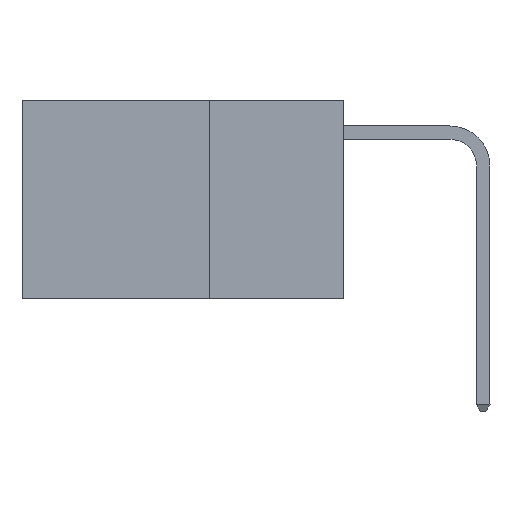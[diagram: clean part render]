
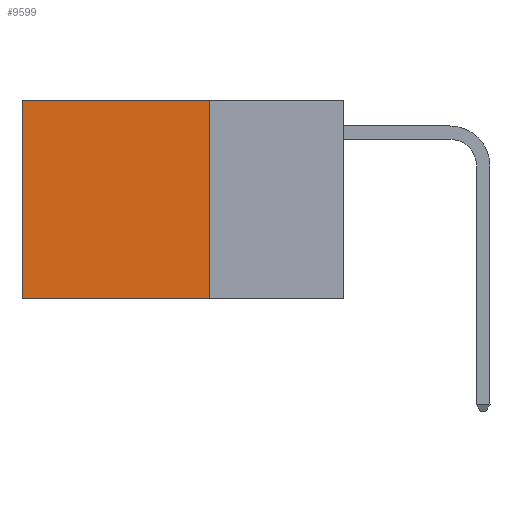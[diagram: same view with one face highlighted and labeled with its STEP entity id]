
A CAD part, left-side view. The second image highlights one B-rep face of the part: STEP entity #9599.
In plain terms, the highlighted planar face has unit normal (-1, 0, 0).
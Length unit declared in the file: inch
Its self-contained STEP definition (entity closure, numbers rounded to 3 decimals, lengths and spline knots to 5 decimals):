
#160 = DIRECTION ( 'NONE',  ( 1., 0., 0. ) ) ;
#245 = VERTEX_POINT ( 'NONE', #9115 ) ;
#525 = CARTESIAN_POINT ( 'NONE',  ( 0.2625, 0.25, -0.37 ) ) ;
#657 = LINE ( 'NONE', #6337, #13990 ) ;
#800 = ORIENTED_EDGE ( 'NONE', *, *, #7438, .F. ) ;
#882 = VECTOR ( 'NONE', #3667, 39.37008 ) ;
#1058 = LINE ( 'NONE', #10226, #7920 ) ;
#1060 = VERTEX_POINT ( 'NONE', #13839 ) ;
#1186 = CARTESIAN_POINT ( 'NONE',  ( 0.2625, 0.6, -0.37 ) ) ;
#1556 = ORIENTED_EDGE ( 'NONE', *, *, #12835, .F. ) ;
#3667 = DIRECTION ( 'NONE',  ( 0., 0., -1. ) ) ;
#4358 = ORIENTED_EDGE ( 'NONE', *, *, #8555, .T. ) ;
#4891 = AXIS2_PLACEMENT_3D ( 'NONE', #8373, #160, #9716 ) ;
#4965 = VERTEX_POINT ( 'NONE', #1186 ) ;
#6168 = CARTESIAN_POINT ( 'NONE',  ( 0.2625, 0.6, 0. ) ) ;
#6178 = ORIENTED_EDGE ( 'NONE', *, *, #6181, .T. ) ;
#6181 = EDGE_CURVE ( 'NONE', #1060, #12550, #657, .T. ) ;
#6337 = CARTESIAN_POINT ( 'NONE',  ( 0.2625, 0.25, 0. ) ) ;
#6612 = EDGE_LOOP ( 'NONE', ( #4358, #1556, #800, #6178 ) ) ;
#6784 = DIRECTION ( 'NONE',  ( 0., 1., 0. ) ) ;
#6867 = VECTOR ( 'NONE', #14300, 39.37008 ) ;
#7438 = EDGE_CURVE ( 'NONE', #1060, #245, #15545, .T. ) ;
#7524 = DIRECTION ( 'NONE',  ( 0., 0., -1. ) ) ;
#7920 = VECTOR ( 'NONE', #7524, 39.37008 ) ;
#8373 = CARTESIAN_POINT ( 'NONE',  ( 0.2625, 0.25, 0. ) ) ;
#8555 = EDGE_CURVE ( 'NONE', #12550, #4965, #1058, .T. ) ;
#9115 = CARTESIAN_POINT ( 'NONE',  ( 0.2625, 0.25, -0.37 ) ) ;
#9599 = ADVANCED_FACE ( 'NONE', ( #11554 ), #16685, .F. ) ;
#9716 = DIRECTION ( 'NONE',  ( 0., 0., -1. ) ) ;
#10226 = CARTESIAN_POINT ( 'NONE',  ( 0.2625, 0.6, 0. ) ) ;
#10447 = CARTESIAN_POINT ( 'NONE',  ( 0.2625, 0.25, 0. ) ) ;
#11554 = FACE_OUTER_BOUND ( 'NONE', #6612, .T. ) ;
#12550 = VERTEX_POINT ( 'NONE', #6168 ) ;
#12835 = EDGE_CURVE ( 'NONE', #245, #4965, #17906, .T. ) ;
#13839 = CARTESIAN_POINT ( 'NONE',  ( 0.2625, 0.25, 0. ) ) ;
#13990 = VECTOR ( 'NONE', #6784, 39.37008 ) ;
#14300 = DIRECTION ( 'NONE',  ( 0., 1., 0. ) ) ;
#15545 = LINE ( 'NONE', #10447, #882 ) ;
#16685 = PLANE ( 'NONE',  #4891 ) ;
#17906 = LINE ( 'NONE', #525, #6867 ) ;
